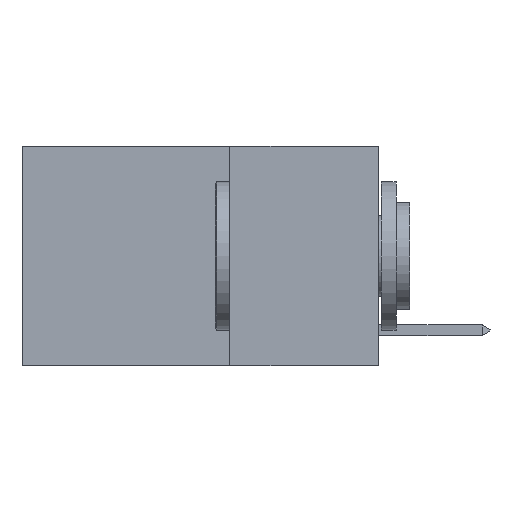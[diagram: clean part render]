
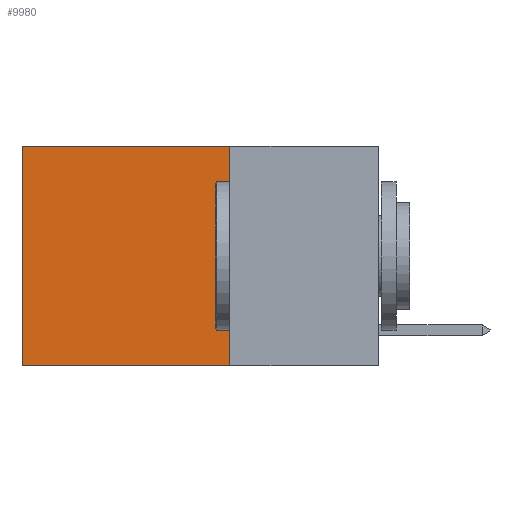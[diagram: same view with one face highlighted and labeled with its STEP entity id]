
A CAD part, left-side view. The second image highlights one B-rep face of the part: STEP entity #9980.
In plain terms, the highlighted planar face has unit normal (-1, 0, 0).
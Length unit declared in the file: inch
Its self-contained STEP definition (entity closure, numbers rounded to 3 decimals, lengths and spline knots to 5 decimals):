
#466 = ORIENTED_EDGE ( 'NONE', *, *, #11423, .F. ) ;
#568 = PLANE ( 'NONE',  #1567 ) ;
#1014 = VECTOR ( 'NONE', #10066, 39.37008 ) ;
#1134 = ORIENTED_EDGE ( 'NONE', *, *, #5978, .T. ) ;
#1235 = CARTESIAN_POINT ( 'NONE',  ( 0.2625, 0.25, -0.37 ) ) ;
#1384 = VECTOR ( 'NONE', #6899, 39.37008 ) ;
#1567 = AXIS2_PLACEMENT_3D ( 'NONE', #16914, #7219, #18495 ) ;
#1945 = CARTESIAN_POINT ( 'NONE',  ( 0.2625, 0.25, 0. ) ) ;
#2348 = VERTEX_POINT ( 'NONE', #12020 ) ;
#3453 = VERTEX_POINT ( 'NONE', #1945 ) ;
#4183 = DIRECTION ( 'NONE',  ( 0., 0., -1. ) ) ;
#5178 = VERTEX_POINT ( 'NONE', #14644 ) ;
#5401 = LINE ( 'NONE', #13295, #1014 ) ;
#5978 = EDGE_CURVE ( 'NONE', #3453, #2348, #13409, .T. ) ;
#6662 = LINE ( 'NONE', #1235, #14767 ) ;
#6899 = DIRECTION ( 'NONE',  ( 0., 1., 0. ) ) ;
#7219 = DIRECTION ( 'NONE',  ( 1., 0., 0. ) ) ;
#8173 = VECTOR ( 'NONE', #4183, 39.37008 ) ;
#9980 = ADVANCED_FACE ( 'NONE', ( #18267 ), #568, .F. ) ;
#10066 = DIRECTION ( 'NONE',  ( 0., 0., -1. ) ) ;
#10470 = EDGE_CURVE ( 'NONE', #2348, #5178, #5401, .T. ) ;
#10731 = CARTESIAN_POINT ( 'NONE',  ( 0.2625, 0.25, 0. ) ) ;
#11077 = DIRECTION ( 'NONE',  ( 0., 1., 0. ) ) ;
#11423 = EDGE_CURVE ( 'NONE', #3453, #15280, #16801, .T. ) ;
#11552 = EDGE_CURVE ( 'NONE', #15280, #5178, #6662, .T. ) ;
#12020 = CARTESIAN_POINT ( 'NONE',  ( 0.2625, 0.6, 0. ) ) ;
#12644 = EDGE_LOOP ( 'NONE', ( #13626, #19453, #466, #1134 ) ) ;
#13295 = CARTESIAN_POINT ( 'NONE',  ( 0.2625, 0.6, 0. ) ) ;
#13307 = CARTESIAN_POINT ( 'NONE',  ( 0.2625, 0.25, -0.37 ) ) ;
#13409 = LINE ( 'NONE', #16594, #1384 ) ;
#13626 = ORIENTED_EDGE ( 'NONE', *, *, #10470, .T. ) ;
#14644 = CARTESIAN_POINT ( 'NONE',  ( 0.2625, 0.6, -0.37 ) ) ;
#14767 = VECTOR ( 'NONE', #11077, 39.37008 ) ;
#15280 = VERTEX_POINT ( 'NONE', #13307 ) ;
#16594 = CARTESIAN_POINT ( 'NONE',  ( 0.2625, 0.25, 0. ) ) ;
#16801 = LINE ( 'NONE', #10731, #8173 ) ;
#16914 = CARTESIAN_POINT ( 'NONE',  ( 0.2625, 0.25, 0. ) ) ;
#18267 = FACE_OUTER_BOUND ( 'NONE', #12644, .T. ) ;
#18495 = DIRECTION ( 'NONE',  ( 0., 0., -1. ) ) ;
#19453 = ORIENTED_EDGE ( 'NONE', *, *, #11552, .F. ) ;
